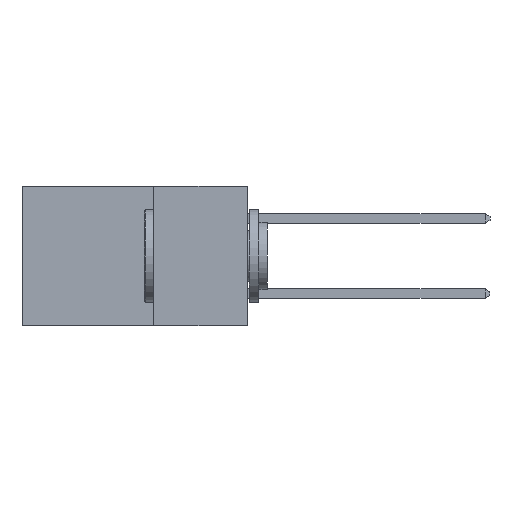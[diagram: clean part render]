
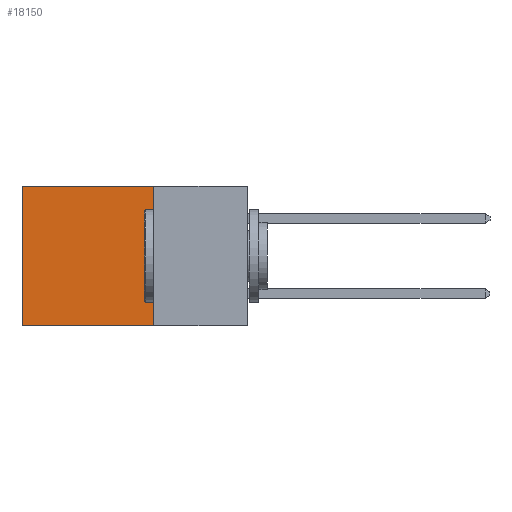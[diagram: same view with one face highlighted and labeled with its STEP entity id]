
A CAD part, left-side view. The second image highlights one B-rep face of the part: STEP entity #18150.
In plain terms, the highlighted planar face has unit normal (-1, 0, 0).
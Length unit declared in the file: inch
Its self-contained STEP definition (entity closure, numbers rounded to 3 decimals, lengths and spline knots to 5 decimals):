
#1250 = VERTEX_POINT ( 'NONE', #24087 ) ;
#2250 = VERTEX_POINT ( 'NONE', #11059 ) ;
#3636 = FACE_OUTER_BOUND ( 'NONE', #27629, .T. ) ;
#6208 = LINE ( 'NONE', #16326, #25476 ) ;
#7197 = VERTEX_POINT ( 'NONE', #14285 ) ;
#8293 = VECTOR ( 'NONE', #10619, 39.37008 ) ;
#9579 = EDGE_CURVE ( 'NONE', #7197, #11290, #29705, .T. ) ;
#10619 = DIRECTION ( 'NONE',  ( 0., 1., 0. ) ) ;
#10863 = CARTESIAN_POINT ( 'NONE',  ( 0.298, 0.25, 0. ) ) ;
#11059 = CARTESIAN_POINT ( 'NONE',  ( 0.298, 0.25, 0. ) ) ;
#11227 = DIRECTION ( 'NONE',  ( 0., 0., -1. ) ) ;
#11290 = VERTEX_POINT ( 'NONE', #11931 ) ;
#11931 = CARTESIAN_POINT ( 'NONE',  ( 0.298, 0.6, -0.37 ) ) ;
#12558 = ORIENTED_EDGE ( 'NONE', *, *, #27389, .T. ) ;
#12608 = DIRECTION ( 'NONE',  ( 0., 0., -1. ) ) ;
#12940 = VECTOR ( 'NONE', #20123, 39.37008 ) ;
#13303 = ORIENTED_EDGE ( 'NONE', *, *, #20044, .F. ) ;
#14285 = CARTESIAN_POINT ( 'NONE',  ( 0.298, 0.6, 0. ) ) ;
#14971 = ORIENTED_EDGE ( 'NONE', *, *, #9579, .T. ) ;
#15239 = CARTESIAN_POINT ( 'NONE',  ( 0.298, 0.25, -0.37 ) ) ;
#16326 = CARTESIAN_POINT ( 'NONE',  ( 0.298, 0.25, 0. ) ) ;
#17563 = AXIS2_PLACEMENT_3D ( 'NONE', #18193, #25140, #11227 ) ;
#18150 = ADVANCED_FACE ( 'NONE', ( #3636 ), #22845, .F. ) ;
#18193 = CARTESIAN_POINT ( 'NONE',  ( 0.298, 0.25, 0. ) ) ;
#18617 = EDGE_CURVE ( 'NONE', #1250, #11290, #26814, .T. ) ;
#20044 = EDGE_CURVE ( 'NONE', #2250, #1250, #23857, .T. ) ;
#20123 = DIRECTION ( 'NONE',  ( 0., 0., -1. ) ) ;
#22845 = PLANE ( 'NONE',  #17563 ) ;
#22940 = VECTOR ( 'NONE', #12608, 39.37008 ) ;
#23857 = LINE ( 'NONE', #10863, #12940 ) ;
#24087 = CARTESIAN_POINT ( 'NONE',  ( 0.298, 0.25, -0.37 ) ) ;
#24224 = CARTESIAN_POINT ( 'NONE',  ( 0.298, 0.6, 0. ) ) ;
#25140 = DIRECTION ( 'NONE',  ( 1., 0., 0. ) ) ;
#25476 = VECTOR ( 'NONE', #25536, 39.37008 ) ;
#25536 = DIRECTION ( 'NONE',  ( 0., 1., 0. ) ) ;
#26814 = LINE ( 'NONE', #15239, #8293 ) ;
#27389 = EDGE_CURVE ( 'NONE', #2250, #7197, #6208, .T. ) ;
#27505 = ORIENTED_EDGE ( 'NONE', *, *, #18617, .F. ) ;
#27629 = EDGE_LOOP ( 'NONE', ( #14971, #27505, #13303, #12558 ) ) ;
#29705 = LINE ( 'NONE', #24224, #22940 ) ;
